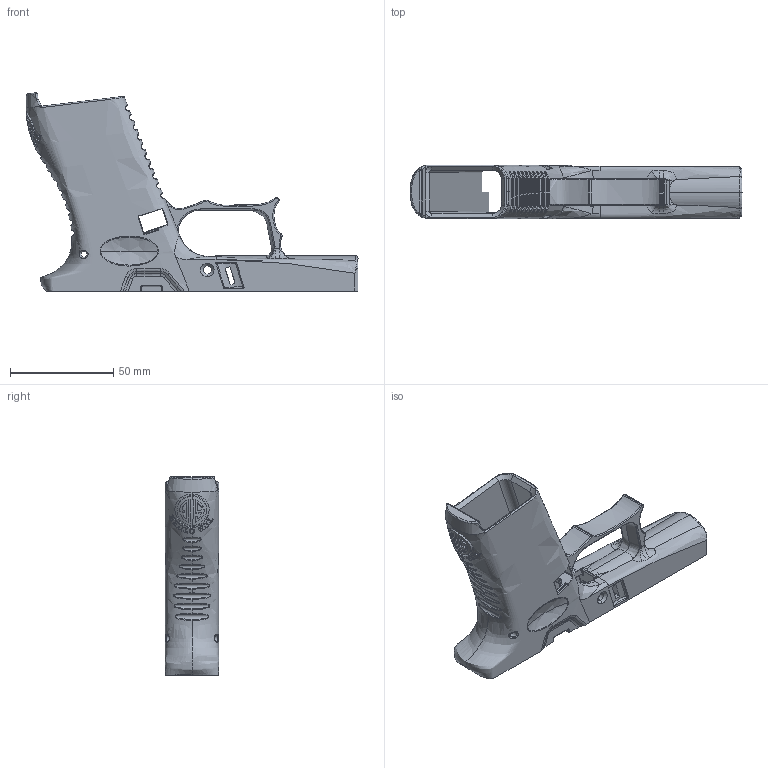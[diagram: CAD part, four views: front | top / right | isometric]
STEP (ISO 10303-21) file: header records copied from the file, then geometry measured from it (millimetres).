
FILE_DESCRIPTION (( 'STEP AP203' ), '1' );
FILE_NAME ('43X SuperSmooth FDM.STEP', '2020-12-17T00:56:27', ( '' ), ( '' ), 'SwSTEP 2.0', 'SolidWorks 2016', '' );
FILE_SCHEMA (( 'CONFIG_CONTROL_DESIGN' ));
Length unit declared in the file: inch
Products named in the file (1): 43X SuperSmooth FDM
Bounding box: 160.56 x 25.9 x 95.92 mm (x, y, z)
Volume: 63433.5 mm3; surface area: 38506.7 mm2
Topology: 1 solids, 1 shells, 1308 faces, 3570 edges, 2234 vertices
Faces by surface type: bspline 464, plane 446, cylinder 358, torus 26, cone 12, sphere 2
Entity records: 84839 total; most frequent: CARTESIAN_POINT 57502, ORIENTED_EDGE 7068, DIRECTION 3680, EDGE_CURVE 3534, VERTEX_POINT 2234, B_SPLINE_CURVE_WITH_KNOTS 1937, AXIS2_PLACEMENT_3D 1344, EDGE_LOOP 1336
